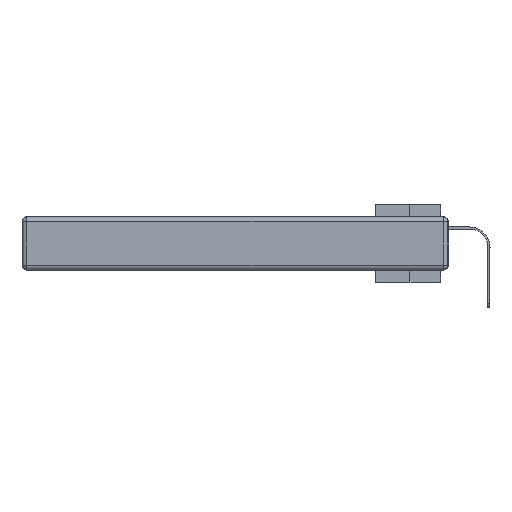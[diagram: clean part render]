
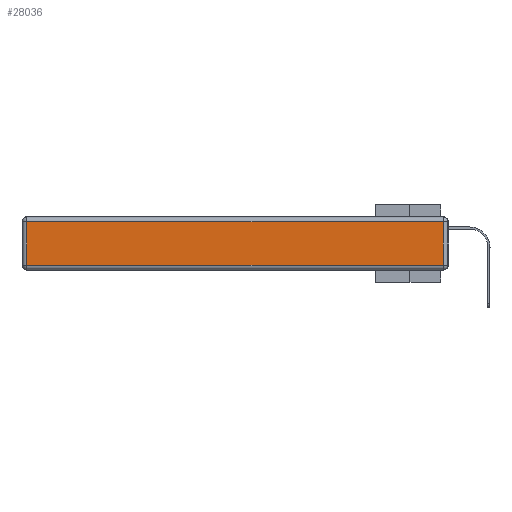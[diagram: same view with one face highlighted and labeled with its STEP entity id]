
A CAD part, left-side view. The second image highlights one B-rep face of the part: STEP entity #28036.
In plain terms, the highlighted planar face has unit normal (-1, 0, 0).
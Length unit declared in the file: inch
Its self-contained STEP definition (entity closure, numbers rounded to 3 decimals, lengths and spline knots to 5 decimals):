
#400 = CARTESIAN_POINT ( 'NONE',  ( 0., 2.72, -0.343 ) ) ;
#2043 = PLANE ( 'NONE',  #26383 ) ;
#3002 = LINE ( 'NONE', #25722, #7695 ) ;
#4220 = ORIENTED_EDGE ( 'NONE', *, *, #31917, .T. ) ;
#4507 = DIRECTION ( 'NONE',  ( -1., 0., 0. ) ) ;
#5028 = ORIENTED_EDGE ( 'NONE', *, *, #27765, .T. ) ;
#6436 = VERTEX_POINT ( 'NONE', #19818 ) ;
#6947 = DIRECTION ( 'NONE',  ( 0., 0., 1. ) ) ;
#7695 = VECTOR ( 'NONE', #13469, 39.37008 ) ;
#8443 = CARTESIAN_POINT ( 'NONE',  ( 0., 2.75, -0.03 ) ) ;
#9330 = ORIENTED_EDGE ( 'NONE', *, *, #21718, .T. ) ;
#10523 = DIRECTION ( 'NONE',  ( 0., 0., -1. ) ) ;
#10731 = DIRECTION ( 'NONE',  ( 0., 1., 0. ) ) ;
#11477 = VECTOR ( 'NONE', #10523, 39.37008 ) ;
#12430 = EDGE_CURVE ( 'NONE', #29664, #13595, #30678, .T. ) ;
#13469 = DIRECTION ( 'NONE',  ( 0., -1., 0. ) ) ;
#13595 = VERTEX_POINT ( 'NONE', #24970 ) ;
#15323 = LINE ( 'NONE', #8443, #20610 ) ;
#15413 = CARTESIAN_POINT ( 'NONE',  ( 0., 2.72, -0.313 ) ) ;
#19818 = CARTESIAN_POINT ( 'NONE',  ( 0., 2.72, -0.03 ) ) ;
#20610 = VECTOR ( 'NONE', #10731, 39.37008 ) ;
#21344 = EDGE_LOOP ( 'NONE', ( #4220, #21955, #5028, #9330 ) ) ;
#21573 = VECTOR ( 'NONE', #30357, 39.37008 ) ;
#21718 = EDGE_CURVE ( 'NONE', #6436, #29949, #22768, .T. ) ;
#21955 = ORIENTED_EDGE ( 'NONE', *, *, #12430, .T. ) ;
#22146 = FACE_OUTER_BOUND ( 'NONE', #21344, .T. ) ;
#22300 = CARTESIAN_POINT ( 'NONE',  ( 0., 0., -0.343 ) ) ;
#22768 = LINE ( 'NONE', #400, #11477 ) ;
#23605 = CARTESIAN_POINT ( 'NONE',  ( 0., 0.03, -0.313 ) ) ;
#24970 = CARTESIAN_POINT ( 'NONE',  ( 0., 0.03, -0.03 ) ) ;
#25722 = CARTESIAN_POINT ( 'NONE',  ( 0., 0., -0.313 ) ) ;
#25781 = CARTESIAN_POINT ( 'NONE',  ( 0., 0.03, -0.343 ) ) ;
#26383 = AXIS2_PLACEMENT_3D ( 'NONE', #22300, #4507, #6947 ) ;
#27765 = EDGE_CURVE ( 'NONE', #13595, #6436, #15323, .T. ) ;
#28036 = ADVANCED_FACE ( 'NONE', ( #22146 ), #2043, .T. ) ;
#29664 = VERTEX_POINT ( 'NONE', #23605 ) ;
#29949 = VERTEX_POINT ( 'NONE', #15413 ) ;
#30357 = DIRECTION ( 'NONE',  ( 0., 0., 1. ) ) ;
#30678 = LINE ( 'NONE', #25781, #21573 ) ;
#31917 = EDGE_CURVE ( 'NONE', #29949, #29664, #3002, .T. ) ;
